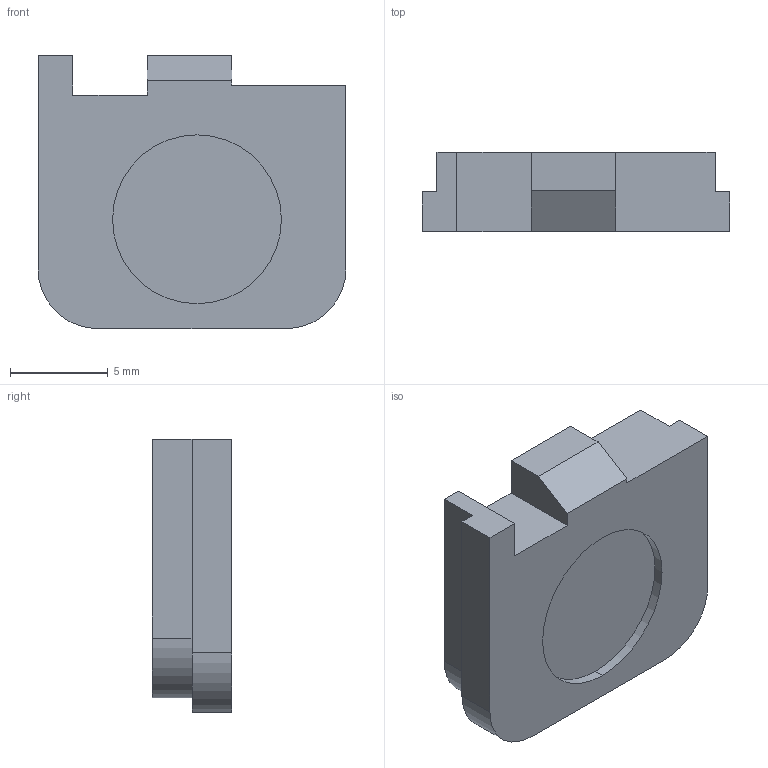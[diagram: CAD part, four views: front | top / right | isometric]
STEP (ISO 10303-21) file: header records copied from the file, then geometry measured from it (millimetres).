
FILE_DESCRIPTION (( 'STEP AP203' ), '1' );
FILE_NAME ('48BPv1.STEP', '2020-08-01T19:57:41', ( '' ), ( '' ), 'SwSTEP 2.0', 'SolidWorks 2020', '' );
FILE_SCHEMA (( 'CONFIG_CONTROL_DESIGN' ));
Length unit declared in the file: inch
Products named in the file (1): 48BPv1
Bounding box: 15.75 x 4.06 x 13.97 mm (x, y, z)
Volume: 711.8 mm3; surface area: 644 mm2
Topology: 1 solids, 1 shells, 24 faces, 63 edges, 42 vertices
Faces by surface type: plane 18, cylinder 6
Entity records: 818 total; most frequent: CARTESIAN_POINT 130, ORIENTED_EDGE 126, DIRECTION 125, EDGE_CURVE 63, VECTOR 51, LINE 51, VERTEX_POINT 42, AXIS2_PLACEMENT_3D 37
